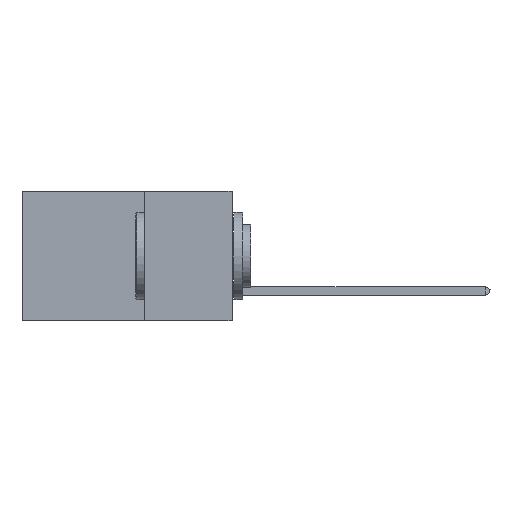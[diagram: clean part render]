
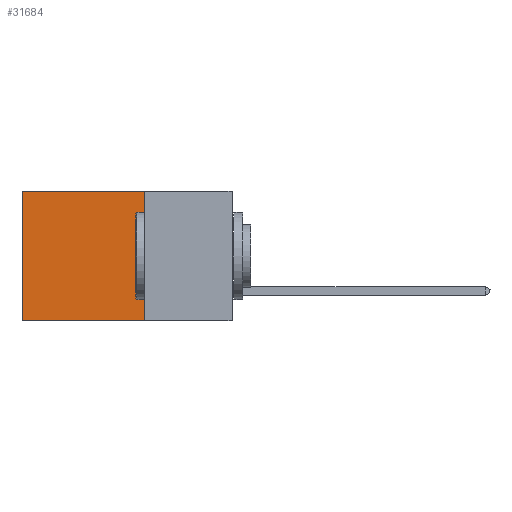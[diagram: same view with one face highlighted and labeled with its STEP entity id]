
A CAD part, left-side view. The second image highlights one B-rep face of the part: STEP entity #31684.
In plain terms, the highlighted planar face has unit normal (-1, 0, 0).
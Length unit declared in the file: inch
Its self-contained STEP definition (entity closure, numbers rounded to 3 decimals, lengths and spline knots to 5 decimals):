
#544 = ORIENTED_EDGE ( 'NONE', *, *, #15803, .F. ) ;
#547 = VECTOR ( 'NONE', #29538, 39.37008 ) ;
#894 = CARTESIAN_POINT ( 'NONE',  ( 0.2875, 0.6, 0. ) ) ;
#1842 = CARTESIAN_POINT ( 'NONE',  ( 0.2875, 0.25, 0. ) ) ;
#2757 = VERTEX_POINT ( 'NONE', #6392 ) ;
#3718 = LINE ( 'NONE', #13868, #10838 ) ;
#3874 = CARTESIAN_POINT ( 'NONE',  ( 0.2875, 0.25, -0.37 ) ) ;
#4031 = LINE ( 'NONE', #1842, #4854 ) ;
#4854 = VECTOR ( 'NONE', #35932, 39.37008 ) ;
#5493 = VERTEX_POINT ( 'NONE', #3874 ) ;
#6023 = DIRECTION ( 'NONE',  ( 1., 0., 0. ) ) ;
#6184 = ORIENTED_EDGE ( 'NONE', *, *, #22237, .T. ) ;
#6392 = CARTESIAN_POINT ( 'NONE',  ( 0.2875, 0.6, -0.37 ) ) ;
#6661 = LINE ( 'NONE', #894, #32580 ) ;
#6751 = ORIENTED_EDGE ( 'NONE', *, *, #26235, .T. ) ;
#7659 = VERTEX_POINT ( 'NONE', #16541 ) ;
#8887 = PLANE ( 'NONE',  #19724 ) ;
#9945 = LINE ( 'NONE', #14939, #547 ) ;
#10099 = ORIENTED_EDGE ( 'NONE', *, *, #20307, .F. ) ;
#10838 = VECTOR ( 'NONE', #16386, 39.37008 ) ;
#13868 = CARTESIAN_POINT ( 'NONE',  ( 0.2875, 0.25, 0. ) ) ;
#14939 = CARTESIAN_POINT ( 'NONE',  ( 0.2875, 0.25, -0.37 ) ) ;
#14979 = DIRECTION ( 'NONE',  ( 0., 0., -1. ) ) ;
#15803 = EDGE_CURVE ( 'NONE', #5493, #2757, #9945, .T. ) ;
#16386 = DIRECTION ( 'NONE',  ( 0., 1., 0. ) ) ;
#16541 = CARTESIAN_POINT ( 'NONE',  ( 0.2875, 0.6, 0. ) ) ;
#17491 = CARTESIAN_POINT ( 'NONE',  ( 0.2875, 0.25, 0. ) ) ;
#19724 = AXIS2_PLACEMENT_3D ( 'NONE', #17491, #6023, #33879 ) ;
#20243 = VERTEX_POINT ( 'NONE', #30278 ) ;
#20307 = EDGE_CURVE ( 'NONE', #20243, #5493, #4031, .T. ) ;
#22237 = EDGE_CURVE ( 'NONE', #7659, #2757, #6661, .T. ) ;
#24686 = FACE_OUTER_BOUND ( 'NONE', #33839, .T. ) ;
#26235 = EDGE_CURVE ( 'NONE', #20243, #7659, #3718, .T. ) ;
#29538 = DIRECTION ( 'NONE',  ( 0., 1., 0. ) ) ;
#30278 = CARTESIAN_POINT ( 'NONE',  ( 0.2875, 0.25, 0. ) ) ;
#31684 = ADVANCED_FACE ( 'NONE', ( #24686 ), #8887, .F. ) ;
#32580 = VECTOR ( 'NONE', #14979, 39.37008 ) ;
#33839 = EDGE_LOOP ( 'NONE', ( #6184, #544, #10099, #6751 ) ) ;
#33879 = DIRECTION ( 'NONE',  ( 0., 0., -1. ) ) ;
#35932 = DIRECTION ( 'NONE',  ( 0., 0., -1. ) ) ;
